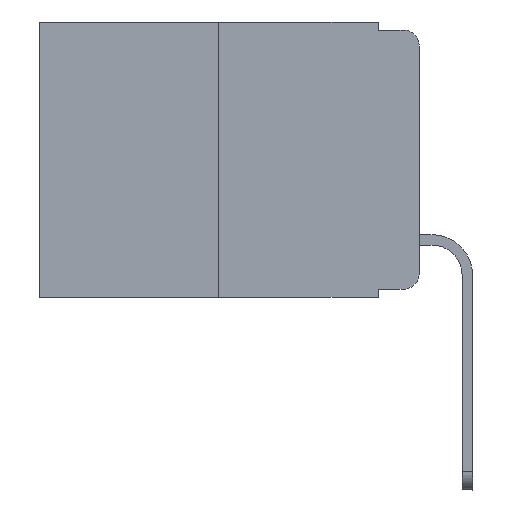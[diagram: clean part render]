
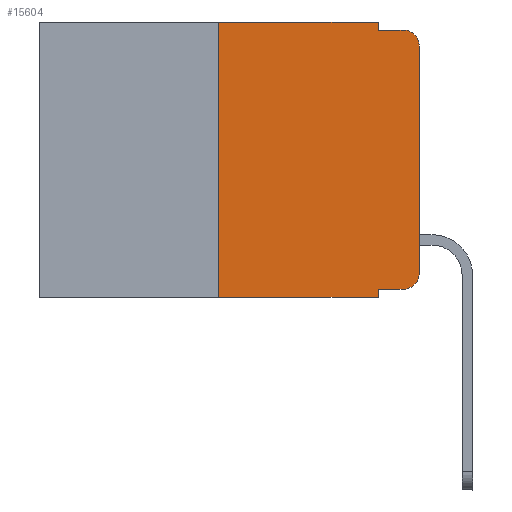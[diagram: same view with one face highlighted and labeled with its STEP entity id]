
A CAD part, left-side view. The second image highlights one B-rep face of the part: STEP entity #15604.
In plain terms, the highlighted planar face has unit normal (-1, 0, 0).
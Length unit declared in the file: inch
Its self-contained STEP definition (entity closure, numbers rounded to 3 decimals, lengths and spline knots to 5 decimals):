
#355 = CARTESIAN_POINT ( 'NONE',  ( 0., 0.25, 0. ) ) ;
#868 = LINE ( 'NONE', #9408, #15470 ) ;
#986 = CARTESIAN_POINT ( 'NONE',  ( 0., 0.02, -0.01 ) ) ;
#1086 = AXIS2_PLACEMENT_3D ( 'NONE', #1419, #3769, #6224 ) ;
#1225 = LINE ( 'NONE', #5939, #9209 ) ;
#1295 = EDGE_CURVE ( 'NONE', #14078, #9052, #13729, .T. ) ;
#1419 = CARTESIAN_POINT ( 'NONE',  ( 0., 0.473, 0. ) ) ;
#1526 = LINE ( 'NONE', #5497, #14713 ) ;
#1833 = CARTESIAN_POINT ( 'NONE',  ( 0., 0.02, -0.313 ) ) ;
#2043 = ORIENTED_EDGE ( 'NONE', *, *, #9899, .T. ) ;
#2069 = EDGE_CURVE ( 'NONE', #10090, #4160, #12426, .T. ) ;
#2545 = EDGE_LOOP ( 'NONE', ( #3613, #2043, #13522, #11411, #13846, #15454, #15941, #5790, #6986, #8763 ) ) ;
#2574 = CIRCLE ( 'NONE', #3860, 0.02 ) ;
#2807 = EDGE_CURVE ( 'NONE', #14078, #3244, #10211, .T. ) ;
#3036 = VECTOR ( 'NONE', #4788, 39.37008 ) ;
#3104 = VECTOR ( 'NONE', #8940, 39.37008 ) ;
#3244 = VERTEX_POINT ( 'NONE', #8605 ) ;
#3343 = VECTOR ( 'NONE', #5230, 39.37008 ) ;
#3377 = EDGE_CURVE ( 'NONE', #3743, #14979, #1526, .T. ) ;
#3470 = CARTESIAN_POINT ( 'NONE',  ( 0., 0.051, -0.333 ) ) ;
#3613 = ORIENTED_EDGE ( 'NONE', *, *, #2069, .T. ) ;
#3652 = DIRECTION ( 'NONE',  ( 0., -1., 0. ) ) ;
#3743 = VERTEX_POINT ( 'NONE', #3470 ) ;
#3769 = DIRECTION ( 'NONE',  ( 1., 0., 0. ) ) ;
#3860 = AXIS2_PLACEMENT_3D ( 'NONE', #15793, #10714, #9334 ) ;
#3903 = CARTESIAN_POINT ( 'NONE',  ( 0., 0., 0. ) ) ;
#4004 = EDGE_CURVE ( 'NONE', #3743, #3244, #868, .T. ) ;
#4068 = CARTESIAN_POINT ( 'NONE',  ( 0., 0., -0.03 ) ) ;
#4160 = VERTEX_POINT ( 'NONE', #4068 ) ;
#4342 = DIRECTION ( 'NONE',  ( -1., 0., 0. ) ) ;
#4376 = VERTEX_POINT ( 'NONE', #986 ) ;
#4788 = DIRECTION ( 'NONE',  ( 0., 0., -1. ) ) ;
#5111 = CARTESIAN_POINT ( 'NONE',  ( 0., 0.051, 0. ) ) ;
#5142 = CIRCLE ( 'NONE', #7724, 0.02 ) ;
#5152 = VECTOR ( 'NONE', #5169, 39.37008 ) ;
#5169 = DIRECTION ( 'NONE',  ( 0., -1., 0. ) ) ;
#5220 = CARTESIAN_POINT ( 'NONE',  ( 0., 0.02, -0.333 ) ) ;
#5230 = DIRECTION ( 'NONE',  ( 0., 0., 1. ) ) ;
#5296 = EDGE_CURVE ( 'NONE', #9052, #11217, #1225, .T. ) ;
#5497 = CARTESIAN_POINT ( 'NONE',  ( 0., 0.051, -0.333 ) ) ;
#5790 = ORIENTED_EDGE ( 'NONE', *, *, #4004, .F. ) ;
#5939 = CARTESIAN_POINT ( 'NONE',  ( 0., 0.473, 0. ) ) ;
#6224 = DIRECTION ( 'NONE',  ( 0., 0., -1. ) ) ;
#6399 = DIRECTION ( 'NONE',  ( 0., -1., 0. ) ) ;
#6986 = ORIENTED_EDGE ( 'NONE', *, *, #3377, .T. ) ;
#7515 = CARTESIAN_POINT ( 'NONE',  ( 0., 0.473, -0.343 ) ) ;
#7724 = AXIS2_PLACEMENT_3D ( 'NONE', #1833, #4342, #9310 ) ;
#8354 = EDGE_CURVE ( 'NONE', #11217, #8738, #10972, .T. ) ;
#8605 = CARTESIAN_POINT ( 'NONE',  ( 0., 0.051, -0.343 ) ) ;
#8738 = VERTEX_POINT ( 'NONE', #12374 ) ;
#8763 = ORIENTED_EDGE ( 'NONE', *, *, #12925, .T. ) ;
#8940 = DIRECTION ( 'NONE',  ( 0., 0., 1. ) ) ;
#9052 = VERTEX_POINT ( 'NONE', #13169 ) ;
#9209 = VECTOR ( 'NONE', #3652, 39.37008 ) ;
#9310 = DIRECTION ( 'NONE',  ( 0., 0., -1. ) ) ;
#9334 = DIRECTION ( 'NONE',  ( 0., 0., -1. ) ) ;
#9408 = CARTESIAN_POINT ( 'NONE',  ( 0., 0.051, 0. ) ) ;
#9642 = FACE_OUTER_BOUND ( 'NONE', #2545, .T. ) ;
#9899 = EDGE_CURVE ( 'NONE', #4160, #4376, #2574, .T. ) ;
#10090 = VERTEX_POINT ( 'NONE', #12865 ) ;
#10211 = LINE ( 'NONE', #7515, #5152 ) ;
#10714 = DIRECTION ( 'NONE',  ( -1., 0., 0. ) ) ;
#10972 = LINE ( 'NONE', #5111, #3036 ) ;
#11015 = CARTESIAN_POINT ( 'NONE',  ( 0., 0.051, -0.01 ) ) ;
#11217 = VERTEX_POINT ( 'NONE', #13767 ) ;
#11411 = ORIENTED_EDGE ( 'NONE', *, *, #8354, .F. ) ;
#11904 = DIRECTION ( 'NONE',  ( 0., 0., -1. ) ) ;
#12374 = CARTESIAN_POINT ( 'NONE',  ( 0., 0.051, -0.01 ) ) ;
#12426 = LINE ( 'NONE', #3903, #3104 ) ;
#12535 = LINE ( 'NONE', #11015, #15561 ) ;
#12865 = CARTESIAN_POINT ( 'NONE',  ( 0., 0., -0.313 ) ) ;
#12925 = EDGE_CURVE ( 'NONE', #14979, #10090, #5142, .T. ) ;
#13169 = CARTESIAN_POINT ( 'NONE',  ( 0., 0.25, 0. ) ) ;
#13522 = ORIENTED_EDGE ( 'NONE', *, *, #15617, .F. ) ;
#13729 = LINE ( 'NONE', #355, #3343 ) ;
#13767 = CARTESIAN_POINT ( 'NONE',  ( 0., 0.051, 0. ) ) ;
#13846 = ORIENTED_EDGE ( 'NONE', *, *, #5296, .F. ) ;
#14076 = CARTESIAN_POINT ( 'NONE',  ( 0., 0.25, -0.343 ) ) ;
#14078 = VERTEX_POINT ( 'NONE', #14076 ) ;
#14565 = PLANE ( 'NONE',  #1086 ) ;
#14713 = VECTOR ( 'NONE', #6399, 39.37008 ) ;
#14979 = VERTEX_POINT ( 'NONE', #5220 ) ;
#15454 = ORIENTED_EDGE ( 'NONE', *, *, #1295, .F. ) ;
#15470 = VECTOR ( 'NONE', #11904, 39.37008 ) ;
#15561 = VECTOR ( 'NONE', #16024, 39.37008 ) ;
#15604 = ADVANCED_FACE ( 'NONE', ( #9642 ), #14565, .F. ) ;
#15617 = EDGE_CURVE ( 'NONE', #8738, #4376, #12535, .T. ) ;
#15793 = CARTESIAN_POINT ( 'NONE',  ( 0., 0.02, -0.03 ) ) ;
#15941 = ORIENTED_EDGE ( 'NONE', *, *, #2807, .T. ) ;
#16024 = DIRECTION ( 'NONE',  ( 0., -1., 0. ) ) ;
